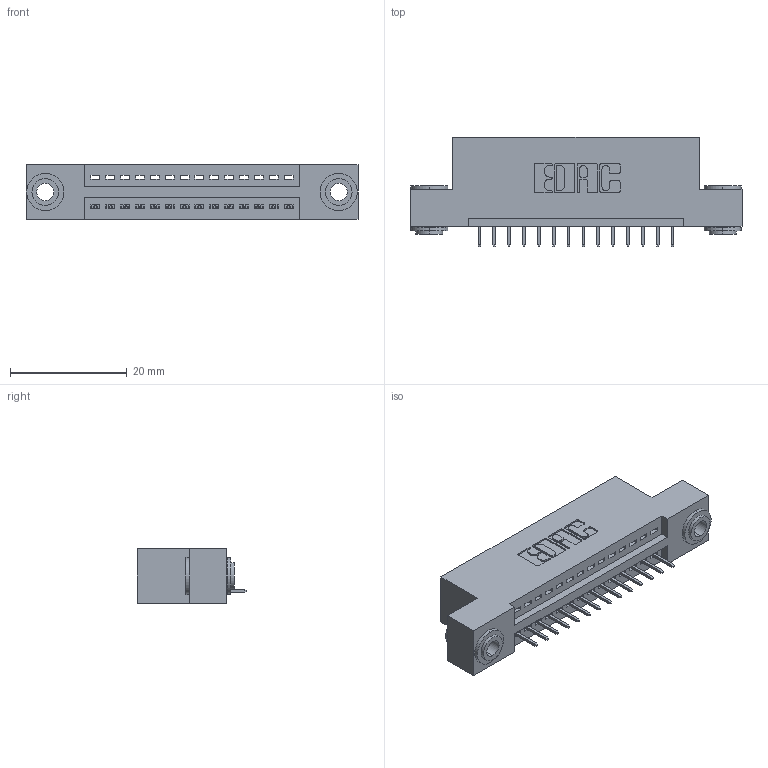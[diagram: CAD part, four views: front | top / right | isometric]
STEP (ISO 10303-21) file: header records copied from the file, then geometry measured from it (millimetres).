
FILE_DESCRIPTION (( 'STEP AP203' ), '1' );
FILE_NAME ('895-014-525-103.STEP', '2020-09-25T03:11:15', ( '' ), ( '' ), 'SwSTEP 2.0', 'SolidWorks 2020', '' );
FILE_SCHEMA (( 'CONFIG_CONTROL_DESIGN' ));
Length unit declared in the file: inch
Products named in the file (4): 845 Part_Flush Mounting Lugs - 0.156 Dia-TH; 895-014-525-103; 345-250-002_345-250-002-102; 345-292-001_345-293-125
Assembly tree (17 placements, depth 2):
  895-014-525-103
    845 Part_Flush Mounting Lugs - 0.156 Dia-TH
    345-292-001_345-293-125  x14
    345-250-002_345-250-002-102  x2
Bounding box: 56.77 x 18.72 x 9.4 mm (x, y, z)
Volume: 5124.8 mm3; surface area: 6453.8 mm2
Topology: 17 solids, 17 shells, 1032 faces, 2937 edges, 1898 vertices
Faces by surface type: plane 734, cylinder 290, cone 8
Entity records: 15030 total; most frequent: CARTESIAN_POINT 2581, ORIENTED_EDGE 2522, DIRECTION 2327, EDGE_CURVE 1261, LINE 1053, VECTOR 1053, VERTEX_POINT 834, AXIS2_PLACEMENT_3D 637
